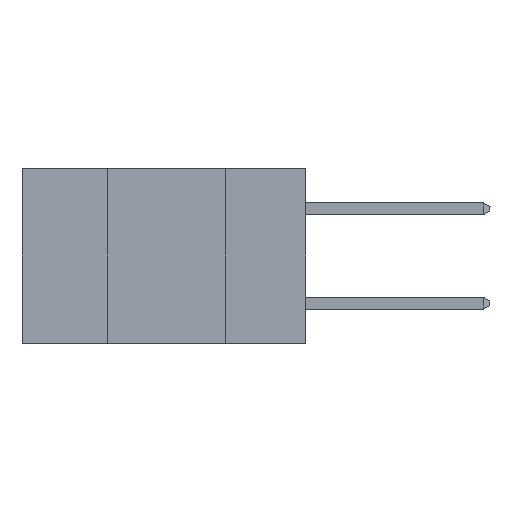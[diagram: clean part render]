
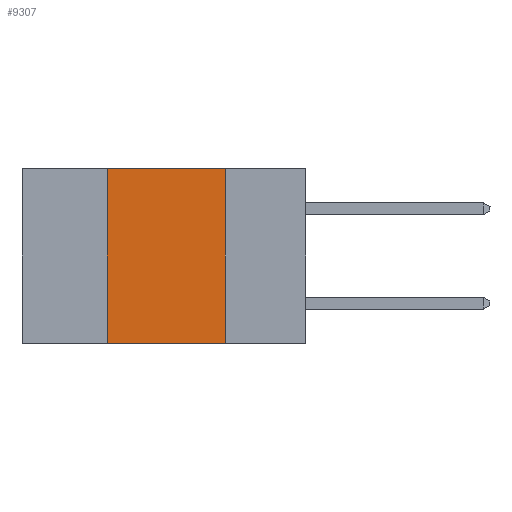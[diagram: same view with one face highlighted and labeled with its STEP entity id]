
A CAD part, left-side view. The second image highlights one B-rep face of the part: STEP entity #9307.
In plain terms, the highlighted planar face has unit normal (-1, 0, 0).
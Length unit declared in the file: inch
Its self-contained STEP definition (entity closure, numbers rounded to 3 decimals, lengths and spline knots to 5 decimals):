
#337 = DIRECTION ( 'NONE',  ( 0., -1., 0. ) ) ;
#1251 = VECTOR ( 'NONE', #24105, 39.37008 ) ;
#1636 = CARTESIAN_POINT ( 'NONE',  ( 0., 0.42, 0. ) ) ;
#2296 = EDGE_CURVE ( 'NONE', #5226, #20104, #7829, .T. ) ;
#4415 = ORIENTED_EDGE ( 'NONE', *, *, #29788, .T. ) ;
#4498 = DIRECTION ( 'NONE',  ( 0., 0., 1. ) ) ;
#5226 = VERTEX_POINT ( 'NONE', #27955 ) ;
#5468 = VECTOR ( 'NONE', #337, 39.37008 ) ;
#6221 = LINE ( 'NONE', #14996, #5468 ) ;
#6470 = EDGE_CURVE ( 'NONE', #23872, #17753, #28708, .T. ) ;
#7829 = LINE ( 'NONE', #27128, #1251 ) ;
#9256 = LINE ( 'NONE', #18972, #29332 ) ;
#9307 = ADVANCED_FACE ( 'NONE', ( #11735 ), #25271, .F. ) ;
#9407 = CARTESIAN_POINT ( 'NONE',  ( 0., 0.42, 0. ) ) ;
#11635 = DIRECTION ( 'NONE',  ( 0., -1., 0. ) ) ;
#11735 = FACE_OUTER_BOUND ( 'NONE', #19062, .T. ) ;
#12134 = ORIENTED_EDGE ( 'NONE', *, *, #6470, .F. ) ;
#13664 = ORIENTED_EDGE ( 'NONE', *, *, #28795, .F. ) ;
#14996 = CARTESIAN_POINT ( 'NONE',  ( 0., 0.6, -0.37 ) ) ;
#17468 = CARTESIAN_POINT ( 'NONE',  ( 0., 0.42, -0.37 ) ) ;
#17753 = VERTEX_POINT ( 'NONE', #9407 ) ;
#18972 = CARTESIAN_POINT ( 'NONE',  ( 0., 0.6, 0. ) ) ;
#19062 = EDGE_LOOP ( 'NONE', ( #20131, #13664, #12134, #4415 ) ) ;
#20104 = VERTEX_POINT ( 'NONE', #29963 ) ;
#20131 = ORIENTED_EDGE ( 'NONE', *, *, #2296, .F. ) ;
#21590 = VECTOR ( 'NONE', #4498, 39.37008 ) ;
#23872 = VERTEX_POINT ( 'NONE', #17468 ) ;
#24105 = DIRECTION ( 'NONE',  ( 0., 0., -1. ) ) ;
#24743 = AXIS2_PLACEMENT_3D ( 'NONE', #25676, #25127, #24861 ) ;
#24861 = DIRECTION ( 'NONE',  ( 0., 0., -1. ) ) ;
#25127 = DIRECTION ( 'NONE',  ( 1., 0., 0. ) ) ;
#25271 = PLANE ( 'NONE',  #24743 ) ;
#25676 = CARTESIAN_POINT ( 'NONE',  ( 0., 0.6, 0. ) ) ;
#27128 = CARTESIAN_POINT ( 'NONE',  ( 0., 0.17, 0. ) ) ;
#27955 = CARTESIAN_POINT ( 'NONE',  ( 0., 0.17, 0. ) ) ;
#28708 = LINE ( 'NONE', #1636, #21590 ) ;
#28795 = EDGE_CURVE ( 'NONE', #17753, #5226, #9256, .T. ) ;
#29332 = VECTOR ( 'NONE', #11635, 39.37008 ) ;
#29788 = EDGE_CURVE ( 'NONE', #23872, #20104, #6221, .T. ) ;
#29963 = CARTESIAN_POINT ( 'NONE',  ( 0., 0.17, -0.37 ) ) ;
